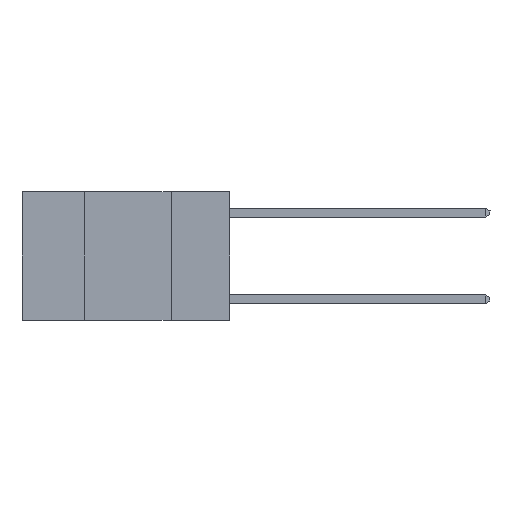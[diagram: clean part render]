
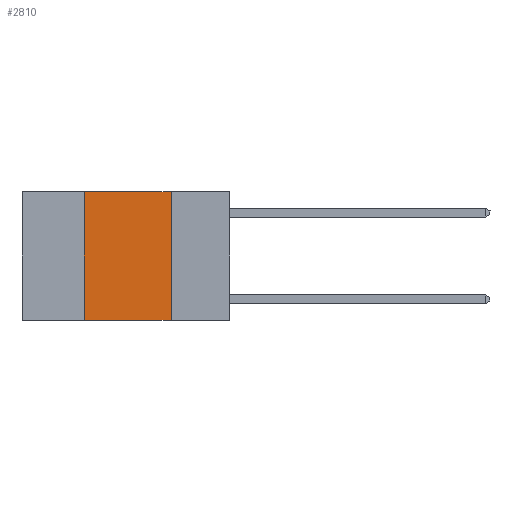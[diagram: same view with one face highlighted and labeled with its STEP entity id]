
A CAD part, left-side view. The second image highlights one B-rep face of the part: STEP entity #2810.
In plain terms, the highlighted planar face has unit normal (-1, 0, 0).
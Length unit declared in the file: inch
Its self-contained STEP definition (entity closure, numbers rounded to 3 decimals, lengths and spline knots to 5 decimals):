
#238 = ORIENTED_EDGE ( 'NONE', *, *, #3220, .F. ) ;
#448 = EDGE_CURVE ( 'NONE', #5167, #2039, #5213, .T. ) ;
#512 = VERTEX_POINT ( 'NONE', #4925 ) ;
#706 = LINE ( 'NONE', #2225, #2628 ) ;
#967 = DIRECTION ( 'NONE',  ( 0., -1., 0. ) ) ;
#1016 = VECTOR ( 'NONE', #5825, 39.37008 ) ;
#1187 = CARTESIAN_POINT ( 'NONE',  ( 0., 0.6, 0. ) ) ;
#1439 = CARTESIAN_POINT ( 'NONE',  ( 0., 0.6, -0.37 ) ) ;
#1509 = EDGE_CURVE ( 'NONE', #5167, #512, #6119, .T. ) ;
#1657 = CARTESIAN_POINT ( 'NONE',  ( 0., 0.6, 0. ) ) ;
#1787 = EDGE_LOOP ( 'NONE', ( #238, #7738, #5993, #7493 ) ) ;
#2039 = VERTEX_POINT ( 'NONE', #8532 ) ;
#2225 = CARTESIAN_POINT ( 'NONE',  ( 0., 0.17, 0. ) ) ;
#2260 = DIRECTION ( 'NONE',  ( 0., 0., -1. ) ) ;
#2261 = EDGE_CURVE ( 'NONE', #2039, #8161, #6903, .T. ) ;
#2628 = VECTOR ( 'NONE', #2260, 39.37008 ) ;
#2810 = ADVANCED_FACE ( 'NONE', ( #4932 ), #3296, .F. ) ;
#3220 = EDGE_CURVE ( 'NONE', #8161, #512, #706, .T. ) ;
#3296 = PLANE ( 'NONE',  #5670 ) ;
#3898 = VECTOR ( 'NONE', #8642, 39.37008 ) ;
#4061 = DIRECTION ( 'NONE',  ( 0., 0., -1. ) ) ;
#4925 = CARTESIAN_POINT ( 'NONE',  ( 0., 0.17, -0.37 ) ) ;
#4930 = VECTOR ( 'NONE', #967, 39.37008 ) ;
#4932 = FACE_OUTER_BOUND ( 'NONE', #1787, .T. ) ;
#5167 = VERTEX_POINT ( 'NONE', #8164 ) ;
#5213 = LINE ( 'NONE', #9767, #1016 ) ;
#5670 = AXIS2_PLACEMENT_3D ( 'NONE', #1657, #8577, #4061 ) ;
#5825 = DIRECTION ( 'NONE',  ( 0., 0., 1. ) ) ;
#5993 = ORIENTED_EDGE ( 'NONE', *, *, #448, .F. ) ;
#6119 = LINE ( 'NONE', #1439, #3898 ) ;
#6903 = LINE ( 'NONE', #1187, #4930 ) ;
#7493 = ORIENTED_EDGE ( 'NONE', *, *, #1509, .T. ) ;
#7738 = ORIENTED_EDGE ( 'NONE', *, *, #2261, .F. ) ;
#8161 = VERTEX_POINT ( 'NONE', #9691 ) ;
#8164 = CARTESIAN_POINT ( 'NONE',  ( 0., 0.42, -0.37 ) ) ;
#8532 = CARTESIAN_POINT ( 'NONE',  ( 0., 0.42, 0. ) ) ;
#8577 = DIRECTION ( 'NONE',  ( 1., 0., 0. ) ) ;
#8642 = DIRECTION ( 'NONE',  ( 0., -1., 0. ) ) ;
#9691 = CARTESIAN_POINT ( 'NONE',  ( 0., 0.17, 0. ) ) ;
#9767 = CARTESIAN_POINT ( 'NONE',  ( 0., 0.42, 0. ) ) ;
